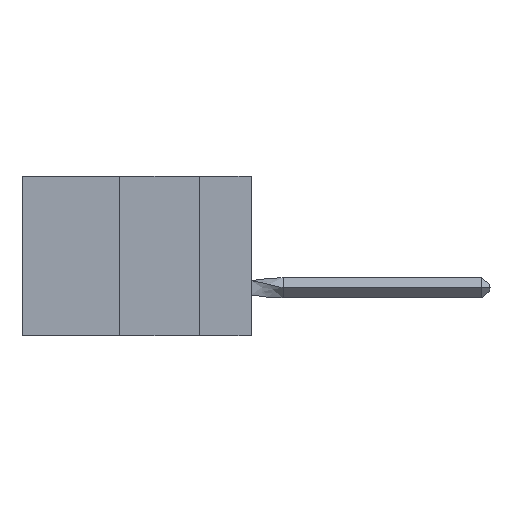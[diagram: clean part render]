
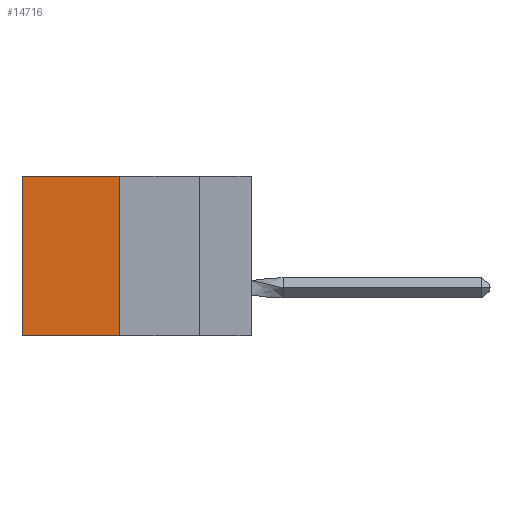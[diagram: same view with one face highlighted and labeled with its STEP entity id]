
A CAD part, left-side view. The second image highlights one B-rep face of the part: STEP entity #14716.
In plain terms, the highlighted planar face has unit normal (-1, 0, 0).
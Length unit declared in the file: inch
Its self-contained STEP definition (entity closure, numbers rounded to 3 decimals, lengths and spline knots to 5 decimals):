
#1103 = VECTOR ( 'NONE', #9448, 39.37008 ) ;
#1593 = ORIENTED_EDGE ( 'NONE', *, *, #12054, .T. ) ;
#2224 = EDGE_CURVE ( 'NONE', #20339, #22010, #18546, .T. ) ;
#2612 = DIRECTION ( 'NONE',  ( 0., 0., -1. ) ) ;
#3506 = CARTESIAN_POINT ( 'NONE',  ( 0.305, 0.72, 0. ) ) ;
#4681 = EDGE_CURVE ( 'NONE', #11798, #14381, #16073, .T. ) ;
#4904 = CARTESIAN_POINT ( 'NONE',  ( 0.305, 0.413, 0. ) ) ;
#6743 = CARTESIAN_POINT ( 'NONE',  ( 0.305, 0.413, -0.5 ) ) ;
#6998 = LINE ( 'NONE', #19054, #21571 ) ;
#6999 = DIRECTION ( 'NONE',  ( 1., 0., 0. ) ) ;
#7943 = ORIENTED_EDGE ( 'NONE', *, *, #4681, .F. ) ;
#8472 = DIRECTION ( 'NONE',  ( 0., 0., -1. ) ) ;
#9448 = DIRECTION ( 'NONE',  ( 0., 1., 0. ) ) ;
#10189 = EDGE_LOOP ( 'NONE', ( #1593, #7943, #18899, #12696 ) ) ;
#11143 = PLANE ( 'NONE',  #26537 ) ;
#11405 = DIRECTION ( 'NONE',  ( 0., 1., 0. ) ) ;
#11798 = VERTEX_POINT ( 'NONE', #20382 ) ;
#12054 = EDGE_CURVE ( 'NONE', #22010, #14381, #6998, .T. ) ;
#12696 = ORIENTED_EDGE ( 'NONE', *, *, #2224, .T. ) ;
#13227 = LINE ( 'NONE', #6743, #14227 ) ;
#14227 = VECTOR ( 'NONE', #2612, 39.37008 ) ;
#14381 = VERTEX_POINT ( 'NONE', #19120 ) ;
#14549 = VECTOR ( 'NONE', #11405, 39.37008 ) ;
#14716 = ADVANCED_FACE ( 'NONE', ( #18414 ), #11143, .F. ) ;
#16073 = LINE ( 'NONE', #17901, #1103 ) ;
#17901 = CARTESIAN_POINT ( 'NONE',  ( 0.305, 0.413, -0.5 ) ) ;
#18414 = FACE_OUTER_BOUND ( 'NONE', #10189, .T. ) ;
#18546 = LINE ( 'NONE', #4904, #14549 ) ;
#18899 = ORIENTED_EDGE ( 'NONE', *, *, #19110, .F. ) ;
#19054 = CARTESIAN_POINT ( 'NONE',  ( 0.305, 0.72, -0.5 ) ) ;
#19110 = EDGE_CURVE ( 'NONE', #20339, #11798, #13227, .T. ) ;
#19120 = CARTESIAN_POINT ( 'NONE',  ( 0.305, 0.72, -0.5 ) ) ;
#20068 = CARTESIAN_POINT ( 'NONE',  ( 0.305, 0.413, -0.5 ) ) ;
#20339 = VERTEX_POINT ( 'NONE', #27301 ) ;
#20382 = CARTESIAN_POINT ( 'NONE',  ( 0.305, 0.413, -0.5 ) ) ;
#21571 = VECTOR ( 'NONE', #8472, 39.37008 ) ;
#22010 = VERTEX_POINT ( 'NONE', #3506 ) ;
#22133 = DIRECTION ( 'NONE',  ( 0., 0., -1. ) ) ;
#26537 = AXIS2_PLACEMENT_3D ( 'NONE', #20068, #6999, #22133 ) ;
#27301 = CARTESIAN_POINT ( 'NONE',  ( 0.305, 0.413, 0. ) ) ;
